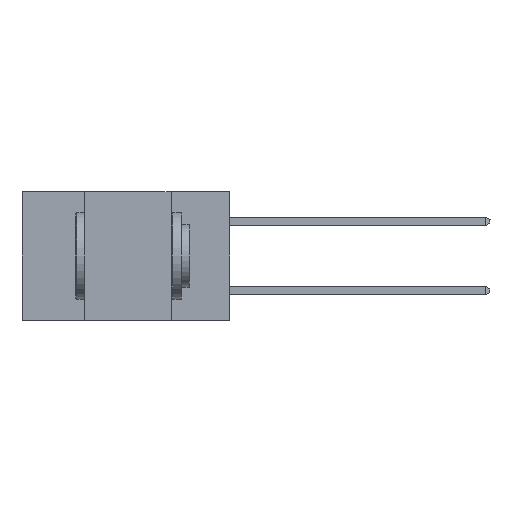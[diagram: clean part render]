
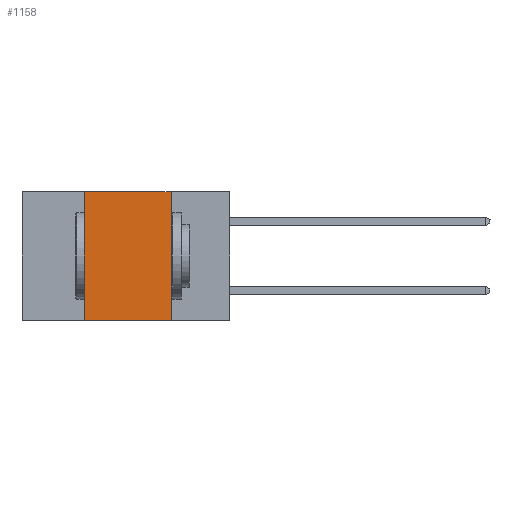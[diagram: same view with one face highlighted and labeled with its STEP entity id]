
A CAD part, left-side view. The second image highlights one B-rep face of the part: STEP entity #1158.
In plain terms, the highlighted planar face has unit normal (-1, 0, 0).
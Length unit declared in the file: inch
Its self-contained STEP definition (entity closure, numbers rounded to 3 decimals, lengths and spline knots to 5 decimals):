
#293 = CARTESIAN_POINT ( 'NONE',  ( 0., 0.42, -0.37 ) ) ;
#467 = DIRECTION ( 'NONE',  ( 0., -1., 0. ) ) ;
#567 = ORIENTED_EDGE ( 'NONE', *, *, #1379, .F. ) ;
#769 = VECTOR ( 'NONE', #6387, 39.37008 ) ;
#1039 = DIRECTION ( 'NONE',  ( 0., 0., -1. ) ) ;
#1122 = LINE ( 'NONE', #8148, #3204 ) ;
#1158 = ADVANCED_FACE ( 'NONE', ( #7235 ), #11377, .F. ) ;
#1280 = VERTEX_POINT ( 'NONE', #3865 ) ;
#1379 = EDGE_CURVE ( 'NONE', #4949, #7076, #8503, .T. ) ;
#2972 = EDGE_CURVE ( 'NONE', #4949, #10091, #5980, .T. ) ;
#2975 = DIRECTION ( 'NONE',  ( 0., -1., 0. ) ) ;
#3204 = VECTOR ( 'NONE', #12349, 39.37008 ) ;
#3865 = CARTESIAN_POINT ( 'NONE',  ( 0., 0.17, 0. ) ) ;
#4412 = CARTESIAN_POINT ( 'NONE',  ( 0., 0.42, -0.37 ) ) ;
#4527 = CARTESIAN_POINT ( 'NONE',  ( 0., 0.17, -0.37 ) ) ;
#4605 = CARTESIAN_POINT ( 'NONE',  ( 0., 0.42, 0. ) ) ;
#4727 = EDGE_CURVE ( 'NONE', #1280, #10091, #1122, .T. ) ;
#4949 = VERTEX_POINT ( 'NONE', #293 ) ;
#5980 = LINE ( 'NONE', #10126, #11426 ) ;
#6387 = DIRECTION ( 'NONE',  ( 0., 0., 1. ) ) ;
#6645 = EDGE_CURVE ( 'NONE', #7076, #1280, #7763, .T. ) ;
#7076 = VERTEX_POINT ( 'NONE', #4605 ) ;
#7092 = ORIENTED_EDGE ( 'NONE', *, *, #2972, .T. ) ;
#7235 = FACE_OUTER_BOUND ( 'NONE', #9088, .T. ) ;
#7763 = LINE ( 'NONE', #11016, #11690 ) ;
#8148 = CARTESIAN_POINT ( 'NONE',  ( 0., 0.17, -0.37 ) ) ;
#8503 = LINE ( 'NONE', #4412, #769 ) ;
#9088 = EDGE_LOOP ( 'NONE', ( #12192, #10523, #567, #7092 ) ) ;
#10091 = VERTEX_POINT ( 'NONE', #4527 ) ;
#10126 = CARTESIAN_POINT ( 'NONE',  ( 0., 0.6, -0.37 ) ) ;
#10357 = CARTESIAN_POINT ( 'NONE',  ( 0., 0.6, 0. ) ) ;
#10424 = DIRECTION ( 'NONE',  ( 1., 0., 0. ) ) ;
#10523 = ORIENTED_EDGE ( 'NONE', *, *, #6645, .F. ) ;
#11016 = CARTESIAN_POINT ( 'NONE',  ( 0., 0.6, 0. ) ) ;
#11377 = PLANE ( 'NONE',  #12228 ) ;
#11426 = VECTOR ( 'NONE', #2975, 39.37008 ) ;
#11690 = VECTOR ( 'NONE', #467, 39.37008 ) ;
#12192 = ORIENTED_EDGE ( 'NONE', *, *, #4727, .F. ) ;
#12228 = AXIS2_PLACEMENT_3D ( 'NONE', #10357, #10424, #1039 ) ;
#12349 = DIRECTION ( 'NONE',  ( 0., 0., -1. ) ) ;
